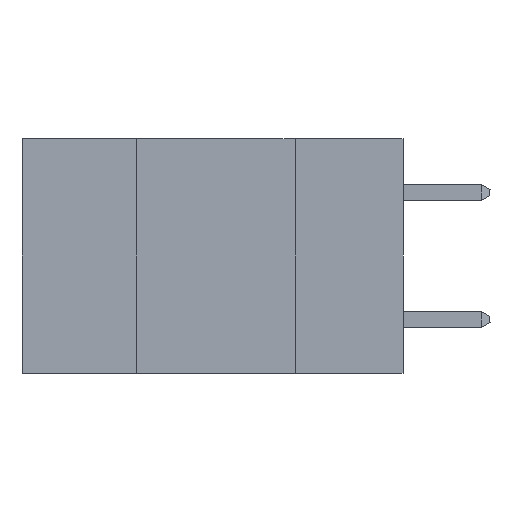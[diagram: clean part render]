
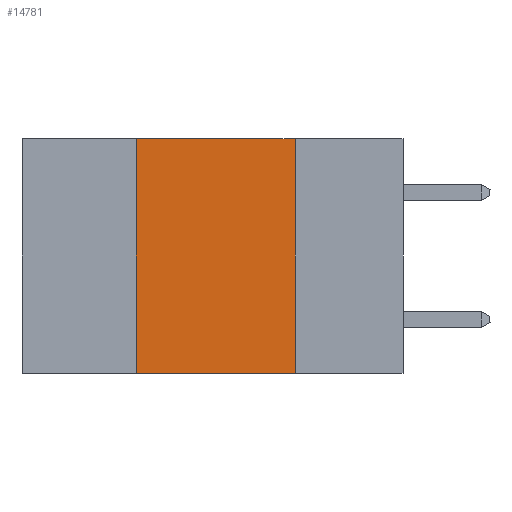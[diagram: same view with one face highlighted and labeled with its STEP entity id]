
A CAD part, left-side view. The second image highlights one B-rep face of the part: STEP entity #14781.
In plain terms, the highlighted planar face has unit normal (-1, 0, 0).
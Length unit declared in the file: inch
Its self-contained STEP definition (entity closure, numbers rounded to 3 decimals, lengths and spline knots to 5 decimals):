
#792 = CARTESIAN_POINT ( 'NONE',  ( 0., 0.17, -0.37 ) ) ;
#1657 = VECTOR ( 'NONE', #4857, 39.37008 ) ;
#2291 = VERTEX_POINT ( 'NONE', #12264 ) ;
#2577 = FACE_OUTER_BOUND ( 'NONE', #8790, .T. ) ;
#3565 = VECTOR ( 'NONE', #21057, 39.37008 ) ;
#3634 = CARTESIAN_POINT ( 'NONE',  ( 0., 0.6, 0. ) ) ;
#3997 = LINE ( 'NONE', #22793, #10150 ) ;
#4513 = VERTEX_POINT ( 'NONE', #7672 ) ;
#4745 = LINE ( 'NONE', #9976, #3565 ) ;
#4857 = DIRECTION ( 'NONE',  ( 0., 0., -1. ) ) ;
#4996 = CARTESIAN_POINT ( 'NONE',  ( 0., 0.42, -0.37 ) ) ;
#5365 = EDGE_CURVE ( 'NONE', #4513, #21113, #7265, .T. ) ;
#5526 = DIRECTION ( 'NONE',  ( 0., 0., -1. ) ) ;
#6911 = EDGE_CURVE ( 'NONE', #2291, #4513, #15335, .T. ) ;
#7180 = EDGE_CURVE ( 'NONE', #15968, #21113, #3997, .T. ) ;
#7265 = LINE ( 'NONE', #15953, #1657 ) ;
#7672 = CARTESIAN_POINT ( 'NONE',  ( 0., 0.17, 0. ) ) ;
#8790 = EDGE_LOOP ( 'NONE', ( #11357, #11036, #10886, #10196 ) ) ;
#9976 = CARTESIAN_POINT ( 'NONE',  ( 0., 0.42, 0. ) ) ;
#10150 = VECTOR ( 'NONE', #11858, 39.37008 ) ;
#10196 = ORIENTED_EDGE ( 'NONE', *, *, #7180, .T. ) ;
#10886 = ORIENTED_EDGE ( 'NONE', *, *, #12713, .F. ) ;
#11036 = ORIENTED_EDGE ( 'NONE', *, *, #6911, .F. ) ;
#11357 = ORIENTED_EDGE ( 'NONE', *, *, #5365, .F. ) ;
#11858 = DIRECTION ( 'NONE',  ( 0., -1., 0. ) ) ;
#12264 = CARTESIAN_POINT ( 'NONE',  ( 0., 0.42, 0. ) ) ;
#12713 = EDGE_CURVE ( 'NONE', #15968, #2291, #4745, .T. ) ;
#14214 = VECTOR ( 'NONE', #16695, 39.37008 ) ;
#14551 = AXIS2_PLACEMENT_3D ( 'NONE', #3634, #16625, #5526 ) ;
#14781 = ADVANCED_FACE ( 'NONE', ( #2577 ), #22049, .F. ) ;
#15335 = LINE ( 'NONE', #22110, #14214 ) ;
#15953 = CARTESIAN_POINT ( 'NONE',  ( 0., 0.17, 0. ) ) ;
#15968 = VERTEX_POINT ( 'NONE', #4996 ) ;
#16625 = DIRECTION ( 'NONE',  ( 1., 0., 0. ) ) ;
#16695 = DIRECTION ( 'NONE',  ( 0., -1., 0. ) ) ;
#21057 = DIRECTION ( 'NONE',  ( 0., 0., 1. ) ) ;
#21113 = VERTEX_POINT ( 'NONE', #792 ) ;
#22049 = PLANE ( 'NONE',  #14551 ) ;
#22110 = CARTESIAN_POINT ( 'NONE',  ( 0., 0.6, 0. ) ) ;
#22793 = CARTESIAN_POINT ( 'NONE',  ( 0., 0.6, -0.37 ) ) ;
